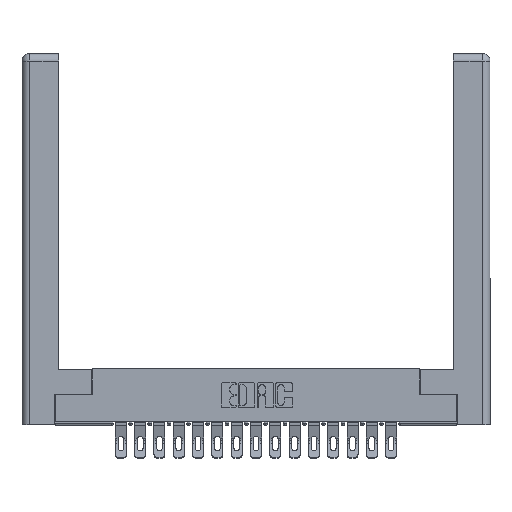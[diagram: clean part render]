
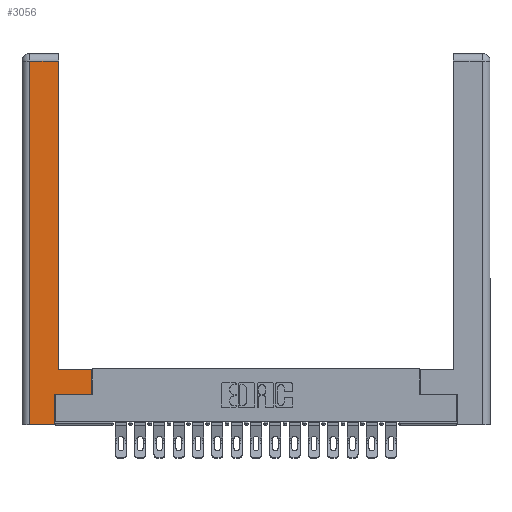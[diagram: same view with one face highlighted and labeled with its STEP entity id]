
A CAD part, top view. The second image highlights one B-rep face of the part: STEP entity #3056.
In plain terms, the highlighted planar face has unit normal (0, 0, 1).
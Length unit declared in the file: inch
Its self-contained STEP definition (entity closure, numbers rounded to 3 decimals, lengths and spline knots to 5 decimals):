
#162 = EDGE_LOOP ( 'NONE', ( #17802, #21140, #12615, #7140, #6822, #19793, #15966, #4023 ) ) ;
#416 = VERTEX_POINT ( 'NONE', #21425 ) ;
#557 = DIRECTION ( 'NONE',  ( 1., 0., 0. ) ) ;
#2007 = VECTOR ( 'NONE', #13348, 39.37008 ) ;
#2023 = CARTESIAN_POINT ( 'NONE',  ( 0.0615, 2.94, 0. ) ) ;
#2423 = VERTEX_POINT ( 'NONE', #21870 ) ;
#2730 = FACE_OUTER_BOUND ( 'NONE', #162, .T. ) ;
#3056 = ADVANCED_FACE ( 'NONE', ( #2730 ), #20065, .F. ) ;
#3845 = DIRECTION ( 'NONE',  ( -1., 0., 0. ) ) ;
#4023 = ORIENTED_EDGE ( 'NONE', *, *, #8013, .T. ) ;
#4174 = CARTESIAN_POINT ( 'NONE',  ( 0.565, 0.45, 0. ) ) ;
#4239 = VERTEX_POINT ( 'NONE', #14033 ) ;
#4245 = LINE ( 'NONE', #13736, #11641 ) ;
#4432 = CARTESIAN_POINT ( 'NONE',  ( 0., 0., 0. ) ) ;
#4851 = CARTESIAN_POINT ( 'NONE',  ( 0.0615, 0., 0. ) ) ;
#5004 = LINE ( 'NONE', #13583, #20716 ) ;
#5013 = EDGE_CURVE ( 'NONE', #4239, #21002, #4245, .T. ) ;
#6454 = DIRECTION ( 'NONE',  ( -1., 0., 0. ) ) ;
#6822 = ORIENTED_EDGE ( 'NONE', *, *, #14916, .T. ) ;
#6896 = DIRECTION ( 'NONE',  ( 1., 0., 0. ) ) ;
#7140 = ORIENTED_EDGE ( 'NONE', *, *, #19762, .T. ) ;
#7486 = CARTESIAN_POINT ( 'NONE',  ( 0.0615, 2.94, 0. ) ) ;
#8013 = EDGE_CURVE ( 'NONE', #21919, #4239, #5004, .T. ) ;
#8021 = EDGE_CURVE ( 'NONE', #19978, #416, #22660, .T. ) ;
#8092 = LINE ( 'NONE', #10999, #16351 ) ;
#8267 = VECTOR ( 'NONE', #16633, 39.37008 ) ;
#8496 = DIRECTION ( 'NONE',  ( 0., 1., 0. ) ) ;
#9103 = LINE ( 'NONE', #13103, #8267 ) ;
#9694 = DIRECTION ( 'NONE',  ( 0., 0., -1. ) ) ;
#10088 = EDGE_CURVE ( 'NONE', #21002, #19978, #16152, .T. ) ;
#10999 = CARTESIAN_POINT ( 'NONE',  ( 0.565, 0.245, 0. ) ) ;
#11624 = VECTOR ( 'NONE', #6896, 39.37008 ) ;
#11641 = VECTOR ( 'NONE', #8496, 39.37008 ) ;
#11846 = VERTEX_POINT ( 'NONE', #19045 ) ;
#12046 = EDGE_CURVE ( 'NONE', #11846, #12637, #8092, .T. ) ;
#12161 = AXIS2_PLACEMENT_3D ( 'NONE', #4432, #9694, #16779 ) ;
#12615 = ORIENTED_EDGE ( 'NONE', *, *, #8021, .T. ) ;
#12637 = VERTEX_POINT ( 'NONE', #16726 ) ;
#13103 = CARTESIAN_POINT ( 'NONE',  ( 0.265, 0.245, 0. ) ) ;
#13348 = DIRECTION ( 'NONE',  ( 0., -1., 0. ) ) ;
#13583 = CARTESIAN_POINT ( 'NONE',  ( 0.295, 0.45, 0. ) ) ;
#13736 = CARTESIAN_POINT ( 'NONE',  ( 0.295, 3., 0. ) ) ;
#14033 = CARTESIAN_POINT ( 'NONE',  ( 0.295, 0.45, 0. ) ) ;
#14510 = VECTOR ( 'NONE', #15205, 39.37008 ) ;
#14916 = EDGE_CURVE ( 'NONE', #2423, #11846, #9103, .T. ) ;
#15205 = DIRECTION ( 'NONE',  ( 0., 1., 0. ) ) ;
#15925 = LINE ( 'NONE', #22311, #14510 ) ;
#15966 = ORIENTED_EDGE ( 'NONE', *, *, #16585, .T. ) ;
#16152 = LINE ( 'NONE', #2023, #19488 ) ;
#16351 = VECTOR ( 'NONE', #557, 39.37008 ) ;
#16585 = EDGE_CURVE ( 'NONE', #12637, #21919, #15925, .T. ) ;
#16633 = DIRECTION ( 'NONE',  ( 0., 1., 0. ) ) ;
#16726 = CARTESIAN_POINT ( 'NONE',  ( 0.565, 0.245, 0. ) ) ;
#16779 = DIRECTION ( 'NONE',  ( -1., 0., 0. ) ) ;
#16900 = LINE ( 'NONE', #22408, #11624 ) ;
#17802 = ORIENTED_EDGE ( 'NONE', *, *, #5013, .T. ) ;
#19045 = CARTESIAN_POINT ( 'NONE',  ( 0.265, 0.245, 0. ) ) ;
#19488 = VECTOR ( 'NONE', #3845, 39.37008 ) ;
#19762 = EDGE_CURVE ( 'NONE', #416, #2423, #16900, .T. ) ;
#19793 = ORIENTED_EDGE ( 'NONE', *, *, #12046, .T. ) ;
#19978 = VERTEX_POINT ( 'NONE', #7486 ) ;
#20065 = PLANE ( 'NONE',  #12161 ) ;
#20716 = VECTOR ( 'NONE', #6454, 39.37008 ) ;
#21002 = VERTEX_POINT ( 'NONE', #22151 ) ;
#21140 = ORIENTED_EDGE ( 'NONE', *, *, #10088, .T. ) ;
#21425 = CARTESIAN_POINT ( 'NONE',  ( 0.0615, 0., 0. ) ) ;
#21870 = CARTESIAN_POINT ( 'NONE',  ( 0.265, 0., 0. ) ) ;
#21919 = VERTEX_POINT ( 'NONE', #4174 ) ;
#22151 = CARTESIAN_POINT ( 'NONE',  ( 0.295, 2.94, 0. ) ) ;
#22311 = CARTESIAN_POINT ( 'NONE',  ( 0.565, 0.45, 0. ) ) ;
#22408 = CARTESIAN_POINT ( 'NONE',  ( 0.265, 0., 0. ) ) ;
#22660 = LINE ( 'NONE', #4851, #2007 ) ;
